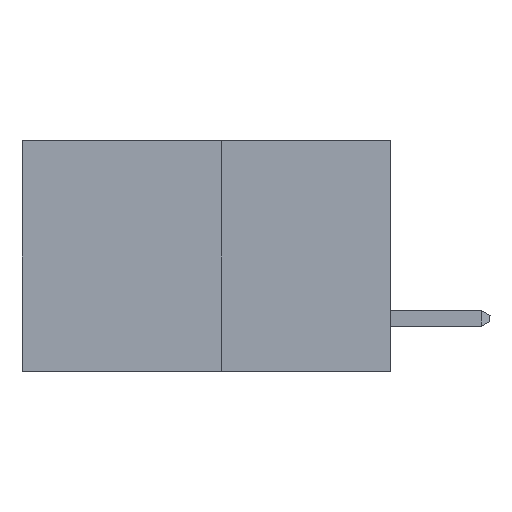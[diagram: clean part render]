
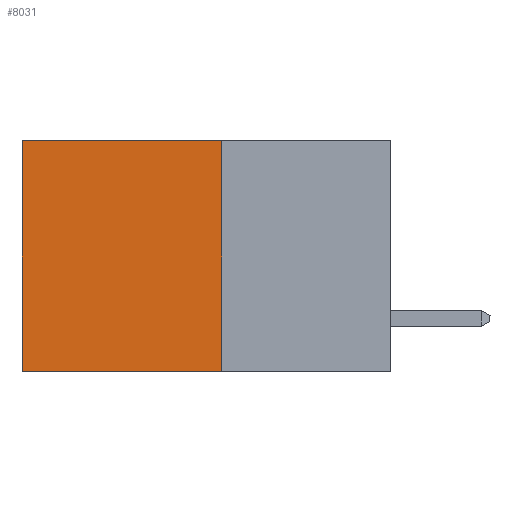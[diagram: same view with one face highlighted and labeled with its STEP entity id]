
A CAD part, left-side view. The second image highlights one B-rep face of the part: STEP entity #8031.
In plain terms, the highlighted planar face has unit normal (-1, 0, 0).
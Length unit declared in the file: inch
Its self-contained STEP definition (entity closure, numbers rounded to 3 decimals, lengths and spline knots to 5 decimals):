
#1084 = FACE_OUTER_BOUND ( 'NONE', #10446, .T. ) ;
#1121 = DIRECTION ( 'NONE',  ( 0., 1., 0. ) ) ;
#2478 = VERTEX_POINT ( 'NONE', #18298 ) ;
#3107 = LINE ( 'NONE', #21204, #7577 ) ;
#3313 = ORIENTED_EDGE ( 'NONE', *, *, #18484, .F. ) ;
#5725 = VECTOR ( 'NONE', #10629, 39.37008 ) ;
#5790 = DIRECTION ( 'NONE',  ( 1., 0., 0. ) ) ;
#5977 = ORIENTED_EDGE ( 'NONE', *, *, #10169, .T. ) ;
#6022 = DIRECTION ( 'NONE',  ( 0., 1., 0. ) ) ;
#6024 = VERTEX_POINT ( 'NONE', #8352 ) ;
#7241 = VECTOR ( 'NONE', #10322, 39.37008 ) ;
#7577 = VECTOR ( 'NONE', #6022, 39.37008 ) ;
#8031 = ADVANCED_FACE ( 'NONE', ( #1084 ), #15239, .F. ) ;
#8302 = LINE ( 'NONE', #23877, #12167 ) ;
#8352 = CARTESIAN_POINT ( 'NONE',  ( 0.277, 0.59, -0.37 ) ) ;
#8360 = CARTESIAN_POINT ( 'NONE',  ( 0.277, 0.27, -0.37 ) ) ;
#10169 = EDGE_CURVE ( 'NONE', #2478, #20075, #3107, .T. ) ;
#10322 = DIRECTION ( 'NONE',  ( 0., 0., -1. ) ) ;
#10446 = EDGE_LOOP ( 'NONE', ( #11252, #3313, #15687, #5977 ) ) ;
#10629 = DIRECTION ( 'NONE',  ( 0., 0., -1. ) ) ;
#11252 = ORIENTED_EDGE ( 'NONE', *, *, #13089, .T. ) ;
#12167 = VECTOR ( 'NONE', #1121, 39.37008 ) ;
#12170 = VERTEX_POINT ( 'NONE', #20970 ) ;
#12299 = LINE ( 'NONE', #8360, #7241 ) ;
#13089 = EDGE_CURVE ( 'NONE', #20075, #6024, #20835, .T. ) ;
#13337 = CARTESIAN_POINT ( 'NONE',  ( 0.277, 0.27, -0.37 ) ) ;
#15239 = PLANE ( 'NONE',  #18539 ) ;
#15687 = ORIENTED_EDGE ( 'NONE', *, *, #21899, .F. ) ;
#18298 = CARTESIAN_POINT ( 'NONE',  ( 0.277, 0.27, 0. ) ) ;
#18484 = EDGE_CURVE ( 'NONE', #12170, #6024, #8302, .T. ) ;
#18539 = AXIS2_PLACEMENT_3D ( 'NONE', #13337, #5790, #19039 ) ;
#19039 = DIRECTION ( 'NONE',  ( 0., 0., -1. ) ) ;
#20075 = VERTEX_POINT ( 'NONE', #23433 ) ;
#20835 = LINE ( 'NONE', #21915, #5725 ) ;
#20970 = CARTESIAN_POINT ( 'NONE',  ( 0.277, 0.27, -0.37 ) ) ;
#21204 = CARTESIAN_POINT ( 'NONE',  ( 0.277, 0.27, 0. ) ) ;
#21899 = EDGE_CURVE ( 'NONE', #2478, #12170, #12299, .T. ) ;
#21915 = CARTESIAN_POINT ( 'NONE',  ( 0.277, 0.59, -0.37 ) ) ;
#23433 = CARTESIAN_POINT ( 'NONE',  ( 0.277, 0.59, 0. ) ) ;
#23877 = CARTESIAN_POINT ( 'NONE',  ( 0.277, 0.27, -0.37 ) ) ;
